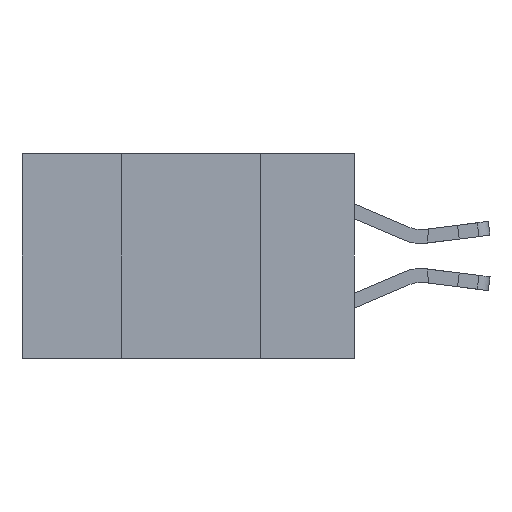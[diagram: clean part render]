
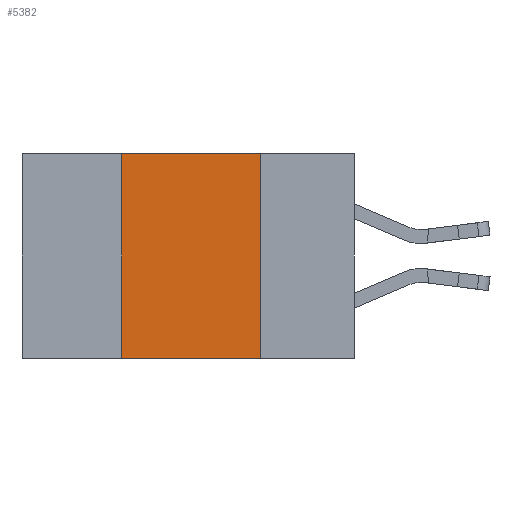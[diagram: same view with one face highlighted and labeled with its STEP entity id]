
A CAD part, left-side view. The second image highlights one B-rep face of the part: STEP entity #5382.
In plain terms, the highlighted planar face has unit normal (-1, 0, 0).
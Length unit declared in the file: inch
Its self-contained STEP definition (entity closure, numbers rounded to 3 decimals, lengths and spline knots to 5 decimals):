
#172 = VECTOR ( 'NONE', #10206, 39.37008 ) ;
#1948 = CARTESIAN_POINT ( 'NONE',  ( 0., 0.42, 0. ) ) ;
#1976 = EDGE_CURVE ( 'NONE', #7016, #12503, #2887, .T. ) ;
#2521 = DIRECTION ( 'NONE',  ( 0., 0., -1. ) ) ;
#2540 = VECTOR ( 'NONE', #4551, 39.37008 ) ;
#2876 = CARTESIAN_POINT ( 'NONE',  ( 0., 0.6, 0. ) ) ;
#2887 = LINE ( 'NONE', #2876, #172 ) ;
#2979 = PLANE ( 'NONE',  #5146 ) ;
#3270 = LINE ( 'NONE', #6692, #5803 ) ;
#3631 = CARTESIAN_POINT ( 'NONE',  ( 0., 0.17, -0.37 ) ) ;
#3797 = CARTESIAN_POINT ( 'NONE',  ( 0., 0.17, 0. ) ) ;
#3979 = DIRECTION ( 'NONE',  ( 0., 0., -1. ) ) ;
#4541 = ORIENTED_EDGE ( 'NONE', *, *, #9156, .F. ) ;
#4551 = DIRECTION ( 'NONE',  ( 0., 0., 1. ) ) ;
#4720 = VERTEX_POINT ( 'NONE', #5662 ) ;
#5146 = AXIS2_PLACEMENT_3D ( 'NONE', #10977, #8981, #3979 ) ;
#5382 = ADVANCED_FACE ( 'NONE', ( #7403 ), #2979, .F. ) ;
#5662 = CARTESIAN_POINT ( 'NONE',  ( 0., 0.42, -0.37 ) ) ;
#5688 = ORIENTED_EDGE ( 'NONE', *, *, #10998, .T. ) ;
#5803 = VECTOR ( 'NONE', #2521, 39.37008 ) ;
#6546 = EDGE_LOOP ( 'NONE', ( #9370, #11519, #4541, #5688 ) ) ;
#6692 = CARTESIAN_POINT ( 'NONE',  ( 0., 0.17, 0. ) ) ;
#7016 = VERTEX_POINT ( 'NONE', #1948 ) ;
#7403 = FACE_OUTER_BOUND ( 'NONE', #6546, .T. ) ;
#7839 = VECTOR ( 'NONE', #7998, 39.37008 ) ;
#7914 = CARTESIAN_POINT ( 'NONE',  ( 0., 0.6, -0.37 ) ) ;
#7998 = DIRECTION ( 'NONE',  ( 0., -1., 0. ) ) ;
#8685 = LINE ( 'NONE', #9485, #2540 ) ;
#8981 = DIRECTION ( 'NONE',  ( 1., 0., 0. ) ) ;
#9156 = EDGE_CURVE ( 'NONE', #4720, #7016, #8685, .T. ) ;
#9283 = VERTEX_POINT ( 'NONE', #3631 ) ;
#9370 = ORIENTED_EDGE ( 'NONE', *, *, #11290, .F. ) ;
#9485 = CARTESIAN_POINT ( 'NONE',  ( 0., 0.42, 0. ) ) ;
#10206 = DIRECTION ( 'NONE',  ( 0., -1., 0. ) ) ;
#10376 = LINE ( 'NONE', #7914, #7839 ) ;
#10977 = CARTESIAN_POINT ( 'NONE',  ( 0., 0.6, 0. ) ) ;
#10998 = EDGE_CURVE ( 'NONE', #4720, #9283, #10376, .T. ) ;
#11290 = EDGE_CURVE ( 'NONE', #12503, #9283, #3270, .T. ) ;
#11519 = ORIENTED_EDGE ( 'NONE', *, *, #1976, .F. ) ;
#12503 = VERTEX_POINT ( 'NONE', #3797 ) ;
